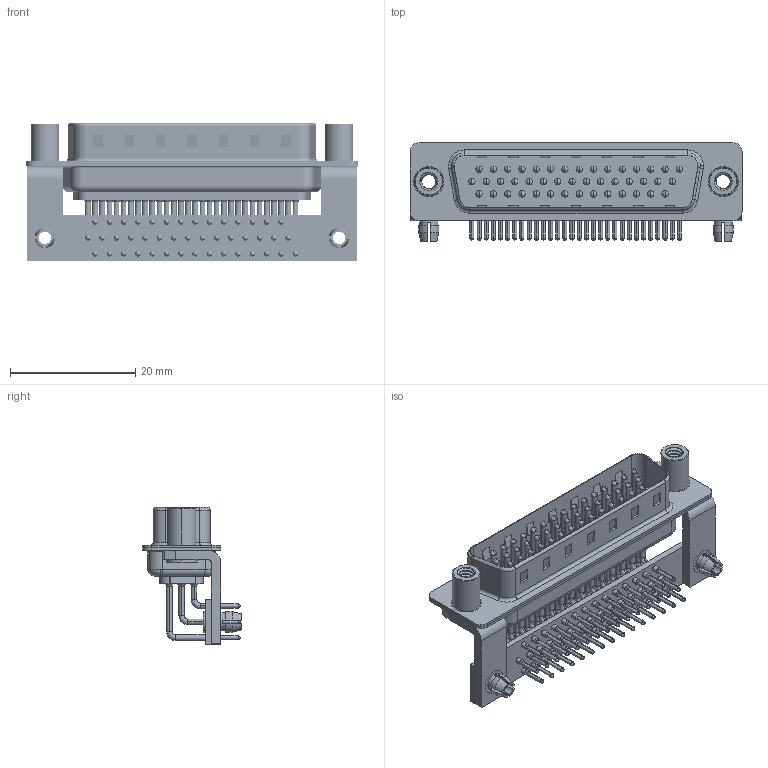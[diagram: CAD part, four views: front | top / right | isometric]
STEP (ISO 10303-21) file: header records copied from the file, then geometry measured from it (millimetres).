
FILE_DESCRIPTION (( 'STEP AP203' ), '1' );
FILE_NAME ('633-M44-663-BN5.STEP', '2018-09-28T01:35:30', ( '' ), ( '' ), 'SwSTEP 2.0', 'SolidWorks 2016', '' );
FILE_SCHEMA (( 'CONFIG_CONTROL_DESIGN' ));
Length unit declared in the file: millimetre
Products named in the file (11): 633M Stabilizer Board_44 Contacts; 633M Housing_44 Contacts; 633M Board Lock; 633M Shell Front_44 Contacts; 633-M44-663-BN5; 633M Shell Rear_44 Contacts; 633M Contact Row 1; 633M Contact Row 2; 633M Contact Row 3; 633M Stabilizer Bracket; 633M 4-40 Threaded Standoff
Assembly tree (54 placements, depth 2):
  633-M44-663-BN5
    633M Housing_44 Contacts
    633M Shell Front_44 Contacts
    633M Shell Rear_44 Contacts
    633M Contact Row 1  x15
    633M Contact Row 2  x15
    633M Contact Row 3  x14
    633M Stabilizer Bracket  x2
    633M 4-40 Threaded Standoff  x2
    633M Stabilizer Board_44 Contacts
    633M Board Lock  x2
Bounding box: 53.05 x 15.8 x 22 mm (x, y, z)
Volume: 3928.5 mm3; surface area: 12174.9 mm2
Topology: 54 solids, 54 shells, 5496 faces, 15405 edges, 10034 vertices
Faces by surface type: plane 3063, cylinder 1905, bspline 270, cone 202, torus 56
Entity records: 41563 total; most frequent: CARTESIAN_POINT 8592, DIRECTION 6741, ORIENTED_EDGE 6134, EDGE_CURVE 3067, AXIS2_PLACEMENT_3D 2537, VERTEX_POINT 2003, VECTOR 1667, LINE 1667
